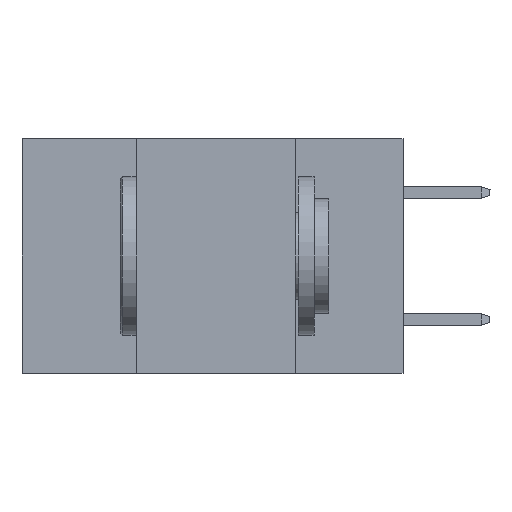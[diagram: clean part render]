
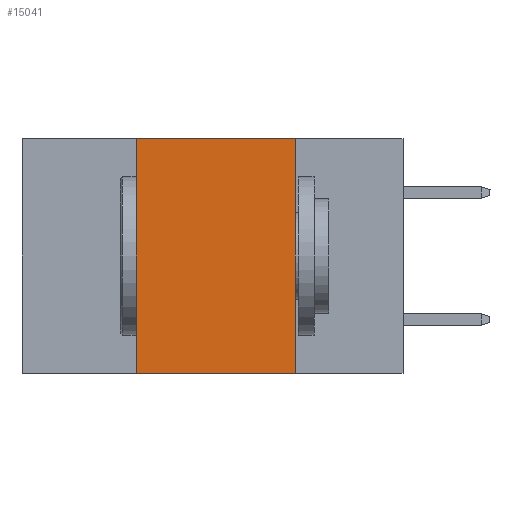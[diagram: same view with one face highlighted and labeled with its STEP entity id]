
A CAD part, left-side view. The second image highlights one B-rep face of the part: STEP entity #15041.
In plain terms, the highlighted planar face has unit normal (-1, 0, 0).
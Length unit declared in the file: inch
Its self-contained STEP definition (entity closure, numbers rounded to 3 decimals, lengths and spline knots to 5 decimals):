
#1206 = LINE ( 'NONE', #33744, #38063 ) ;
#2142 = EDGE_LOOP ( 'NONE', ( #20168, #24236, #10528, #28593 ) ) ;
#3517 = PLANE ( 'NONE',  #16410 ) ;
#3735 = LINE ( 'NONE', #25528, #12536 ) ;
#4256 = VECTOR ( 'NONE', #35565, 39.37008 ) ;
#4272 = LINE ( 'NONE', #29319, #43669 ) ;
#4646 = VERTEX_POINT ( 'NONE', #38433 ) ;
#5177 = DIRECTION ( 'NONE',  ( 0., 0., -1. ) ) ;
#7270 = DIRECTION ( 'NONE',  ( 0., 0., -1. ) ) ;
#8262 = EDGE_CURVE ( 'NONE', #10194, #32183, #1206, .T. ) ;
#10194 = VERTEX_POINT ( 'NONE', #11423 ) ;
#10528 = ORIENTED_EDGE ( 'NONE', *, *, #19388, .F. ) ;
#10790 = CARTESIAN_POINT ( 'NONE',  ( 0., 0.6, 0. ) ) ;
#11423 = CARTESIAN_POINT ( 'NONE',  ( 0., 0.17, 0. ) ) ;
#12536 = VECTOR ( 'NONE', #36277, 39.37008 ) ;
#14263 = VERTEX_POINT ( 'NONE', #33415 ) ;
#15041 = ADVANCED_FACE ( 'NONE', ( #43510 ), #3517, .F. ) ;
#16410 = AXIS2_PLACEMENT_3D ( 'NONE', #10790, #17810, #7270 ) ;
#17810 = DIRECTION ( 'NONE',  ( 1., 0., 0. ) ) ;
#19388 = EDGE_CURVE ( 'NONE', #4646, #14263, #4272, .T. ) ;
#20168 = ORIENTED_EDGE ( 'NONE', *, *, #8262, .F. ) ;
#21314 = CARTESIAN_POINT ( 'NONE',  ( 0., 0.6, -0.37 ) ) ;
#21827 = EDGE_CURVE ( 'NONE', #14263, #10194, #3735, .T. ) ;
#24236 = ORIENTED_EDGE ( 'NONE', *, *, #21827, .F. ) ;
#25528 = CARTESIAN_POINT ( 'NONE',  ( 0., 0.6, 0. ) ) ;
#26707 = CARTESIAN_POINT ( 'NONE',  ( 0., 0.17, -0.37 ) ) ;
#28141 = EDGE_CURVE ( 'NONE', #4646, #32183, #45619, .T. ) ;
#28593 = ORIENTED_EDGE ( 'NONE', *, *, #28141, .T. ) ;
#29319 = CARTESIAN_POINT ( 'NONE',  ( 0., 0.42, 0. ) ) ;
#32183 = VERTEX_POINT ( 'NONE', #26707 ) ;
#33415 = CARTESIAN_POINT ( 'NONE',  ( 0., 0.42, 0. ) ) ;
#33744 = CARTESIAN_POINT ( 'NONE',  ( 0., 0.17, 0. ) ) ;
#35565 = DIRECTION ( 'NONE',  ( 0., -1., 0. ) ) ;
#36277 = DIRECTION ( 'NONE',  ( 0., -1., 0. ) ) ;
#38063 = VECTOR ( 'NONE', #5177, 39.37008 ) ;
#38433 = CARTESIAN_POINT ( 'NONE',  ( 0., 0.42, -0.37 ) ) ;
#43510 = FACE_OUTER_BOUND ( 'NONE', #2142, .T. ) ;
#43556 = DIRECTION ( 'NONE',  ( 0., 0., 1. ) ) ;
#43669 = VECTOR ( 'NONE', #43556, 39.37008 ) ;
#45619 = LINE ( 'NONE', #21314, #4256 ) ;
